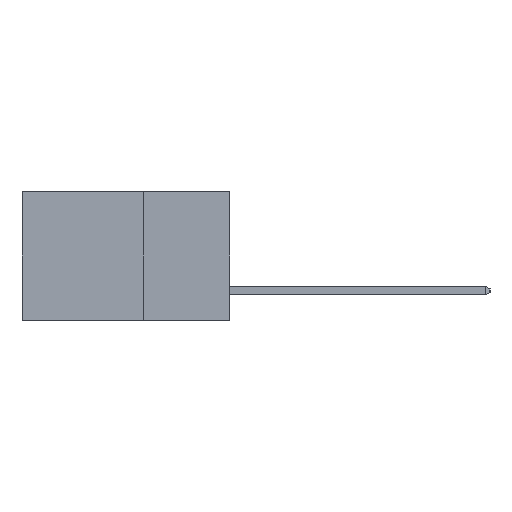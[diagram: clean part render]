
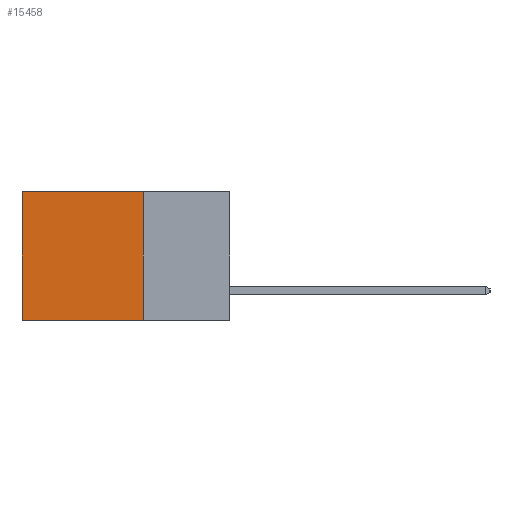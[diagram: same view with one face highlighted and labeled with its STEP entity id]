
A CAD part, left-side view. The second image highlights one B-rep face of the part: STEP entity #15458.
In plain terms, the highlighted planar face has unit normal (-1, 0, 0).
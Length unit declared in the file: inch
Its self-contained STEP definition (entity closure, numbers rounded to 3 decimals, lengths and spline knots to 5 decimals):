
#749 = CARTESIAN_POINT ( 'NONE',  ( 0.298, 0.25, -0.37 ) ) ;
#999 = VECTOR ( 'NONE', #1153, 39.37008 ) ;
#1153 = DIRECTION ( 'NONE',  ( 0., 1., 0. ) ) ;
#1259 = CARTESIAN_POINT ( 'NONE',  ( 0.298, 0.25, -0.37 ) ) ;
#2257 = AXIS2_PLACEMENT_3D ( 'NONE', #11937, #4419, #13203 ) ;
#3788 = VECTOR ( 'NONE', #3987, 39.37008 ) ;
#3987 = DIRECTION ( 'NONE',  ( 0., 0., -1. ) ) ;
#4000 = VERTEX_POINT ( 'NONE', #749 ) ;
#4048 = LINE ( 'NONE', #1259, #999 ) ;
#4372 = CARTESIAN_POINT ( 'NONE',  ( 0.298, 0.6, 0. ) ) ;
#4419 = DIRECTION ( 'NONE',  ( 1., 0., 0. ) ) ;
#4812 = VECTOR ( 'NONE', #10884, 39.37008 ) ;
#5649 = EDGE_CURVE ( 'NONE', #4000, #6201, #4048, .T. ) ;
#5690 = EDGE_CURVE ( 'NONE', #10769, #6201, #10161, .T. ) ;
#6201 = VERTEX_POINT ( 'NONE', #8937 ) ;
#6564 = EDGE_LOOP ( 'NONE', ( #8631, #14610, #15754, #9280 ) ) ;
#6663 = DIRECTION ( 'NONE',  ( 0., 1., 0. ) ) ;
#7452 = VERTEX_POINT ( 'NONE', #13143 ) ;
#8631 = ORIENTED_EDGE ( 'NONE', *, *, #5690, .T. ) ;
#8928 = LINE ( 'NONE', #15438, #12193 ) ;
#8937 = CARTESIAN_POINT ( 'NONE',  ( 0.298, 0.6, -0.37 ) ) ;
#9280 = ORIENTED_EDGE ( 'NONE', *, *, #12770, .T. ) ;
#9380 = FACE_OUTER_BOUND ( 'NONE', #6564, .T. ) ;
#9491 = PLANE ( 'NONE',  #2257 ) ;
#9674 = CARTESIAN_POINT ( 'NONE',  ( 0.298, 0.25, 0. ) ) ;
#10161 = LINE ( 'NONE', #4372, #3788 ) ;
#10769 = VERTEX_POINT ( 'NONE', #15471 ) ;
#10884 = DIRECTION ( 'NONE',  ( 0., 0., -1. ) ) ;
#11937 = CARTESIAN_POINT ( 'NONE',  ( 0.298, 0.25, 0. ) ) ;
#12193 = VECTOR ( 'NONE', #6663, 39.37008 ) ;
#12770 = EDGE_CURVE ( 'NONE', #7452, #10769, #8928, .T. ) ;
#13143 = CARTESIAN_POINT ( 'NONE',  ( 0.298, 0.25, 0. ) ) ;
#13203 = DIRECTION ( 'NONE',  ( 0., 0., -1. ) ) ;
#14610 = ORIENTED_EDGE ( 'NONE', *, *, #5649, .F. ) ;
#14808 = LINE ( 'NONE', #9674, #4812 ) ;
#14890 = EDGE_CURVE ( 'NONE', #7452, #4000, #14808, .T. ) ;
#15438 = CARTESIAN_POINT ( 'NONE',  ( 0.298, 0.25, 0. ) ) ;
#15458 = ADVANCED_FACE ( 'NONE', ( #9380 ), #9491, .F. ) ;
#15471 = CARTESIAN_POINT ( 'NONE',  ( 0.298, 0.6, 0. ) ) ;
#15754 = ORIENTED_EDGE ( 'NONE', *, *, #14890, .F. ) ;
